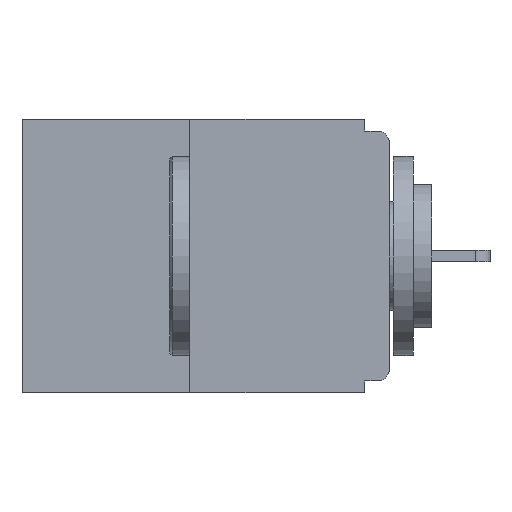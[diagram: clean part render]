
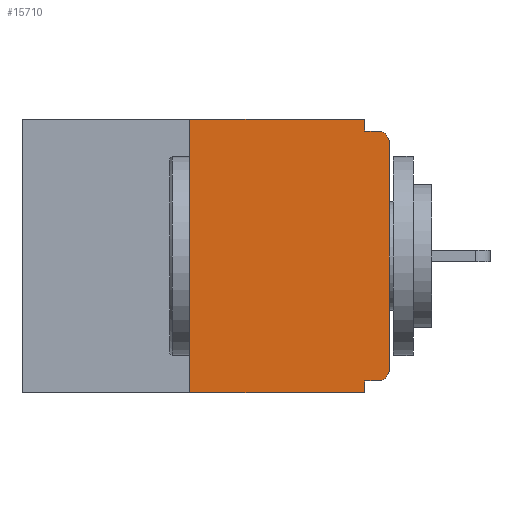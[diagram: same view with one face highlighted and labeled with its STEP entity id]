
A CAD part, left-side view. The second image highlights one B-rep face of the part: STEP entity #15710.
In plain terms, the highlighted planar face has unit normal (-1, 0, 0).
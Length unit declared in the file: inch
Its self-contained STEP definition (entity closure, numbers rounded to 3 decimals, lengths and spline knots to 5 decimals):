
#80 = VECTOR ( 'NONE', #3556, 39.37008 ) ;
#106 = EDGE_CURVE ( 'NONE', #14597, #6635, #15240, .T. ) ;
#530 = CARTESIAN_POINT ( 'NONE',  ( 0., 0.031, -0.343 ) ) ;
#645 = DIRECTION ( 'NONE',  ( 0., -1., 0. ) ) ;
#669 = VECTOR ( 'NONE', #9693, 39.37008 ) ;
#735 = VERTEX_POINT ( 'NONE', #10886 ) ;
#1963 = VERTEX_POINT ( 'NONE', #6756 ) ;
#2174 = CARTESIAN_POINT ( 'NONE',  ( 0., 0.031, -0.343 ) ) ;
#2885 = ORIENTED_EDGE ( 'NONE', *, *, #7124, .T. ) ;
#2951 = CARTESIAN_POINT ( 'NONE',  ( 0., 0.031, 0. ) ) ;
#3528 = EDGE_CURVE ( 'NONE', #10391, #17721, #3799, .T. ) ;
#3556 = DIRECTION ( 'NONE',  ( 0., -1., 0. ) ) ;
#3703 = DIRECTION ( 'NONE',  ( 0., 0., -1. ) ) ;
#3710 = LINE ( 'NONE', #10518, #11181 ) ;
#3799 = LINE ( 'NONE', #8110, #669 ) ;
#3952 = LINE ( 'NONE', #2951, #19208 ) ;
#4292 = VERTEX_POINT ( 'NONE', #530 ) ;
#4637 = LINE ( 'NONE', #11013, #80 ) ;
#4674 = DIRECTION ( 'NONE',  ( 0., 0., -1. ) ) ;
#4984 = ORIENTED_EDGE ( 'NONE', *, *, #16975, .F. ) ;
#5549 = AXIS2_PLACEMENT_3D ( 'NONE', #8939, #8842, #8495 ) ;
#6229 = VERTEX_POINT ( 'NONE', #10614 ) ;
#6635 = VERTEX_POINT ( 'NONE', #9253 ) ;
#6756 = CARTESIAN_POINT ( 'NONE',  ( 0., 0., -0.313 ) ) ;
#6788 = VECTOR ( 'NONE', #645, 39.37008 ) ;
#6792 = CARTESIAN_POINT ( 'NONE',  ( 0., 0.031, 0. ) ) ;
#6859 = ORIENTED_EDGE ( 'NONE', *, *, #19126, .T. ) ;
#6990 = CARTESIAN_POINT ( 'NONE',  ( 0., 0.25, 0. ) ) ;
#6999 = VECTOR ( 'NONE', #8473, 39.37008 ) ;
#7124 = EDGE_CURVE ( 'NONE', #10391, #1963, #13914, .T. ) ;
#7157 = LINE ( 'NONE', #9190, #17607 ) ;
#7274 = CARTESIAN_POINT ( 'NONE',  ( 0., 0.031, -0.328 ) ) ;
#7307 = ORIENTED_EDGE ( 'NONE', *, *, #106, .T. ) ;
#7962 = EDGE_LOOP ( 'NONE', ( #16405, #4984, #13426, #13890, #14345, #2885, #6859, #7307, #15253, #19100 ) ) ;
#8110 = CARTESIAN_POINT ( 'NONE',  ( 0., 0., -0.328 ) ) ;
#8422 = AXIS2_PLACEMENT_3D ( 'NONE', #12131, #13645, #4674 ) ;
#8466 = VERTEX_POINT ( 'NONE', #6792 ) ;
#8473 = DIRECTION ( 'NONE',  ( 0., 0., 1. ) ) ;
#8495 = DIRECTION ( 'NONE',  ( 0., 0., -1. ) ) ;
#8534 = CARTESIAN_POINT ( 'NONE',  ( 0., 0.015, -0.328 ) ) ;
#8842 = DIRECTION ( 'NONE',  ( -1., 0., 0. ) ) ;
#8939 = CARTESIAN_POINT ( 'NONE',  ( 0., 0.015, -0.03 ) ) ;
#9190 = CARTESIAN_POINT ( 'NONE',  ( 0., 0., 0. ) ) ;
#9253 = CARTESIAN_POINT ( 'NONE',  ( 0., 0.015, -0.015 ) ) ;
#9652 = CARTESIAN_POINT ( 'NONE',  ( 0., 0., -0.015 ) ) ;
#9693 = DIRECTION ( 'NONE',  ( 0., 1., 0. ) ) ;
#10391 = VERTEX_POINT ( 'NONE', #8534 ) ;
#10518 = CARTESIAN_POINT ( 'NONE',  ( 0., 0.46, -0.343 ) ) ;
#10614 = CARTESIAN_POINT ( 'NONE',  ( 0., 0.25, 0. ) ) ;
#10733 = CARTESIAN_POINT ( 'NONE',  ( 0., 0.031, -0.015 ) ) ;
#10886 = CARTESIAN_POINT ( 'NONE',  ( 0., 0.25, -0.343 ) ) ;
#11011 = LINE ( 'NONE', #6990, #6999 ) ;
#11013 = CARTESIAN_POINT ( 'NONE',  ( 0., 0.46, 0. ) ) ;
#11181 = VECTOR ( 'NONE', #16424, 39.37008 ) ;
#11700 = VECTOR ( 'NONE', #3703, 39.37008 ) ;
#11924 = EDGE_CURVE ( 'NONE', #17721, #4292, #16095, .T. ) ;
#12131 = CARTESIAN_POINT ( 'NONE',  ( 0., 0.46, 0. ) ) ;
#13426 = ORIENTED_EDGE ( 'NONE', *, *, #19044, .T. ) ;
#13645 = DIRECTION ( 'NONE',  ( 1., 0., 0. ) ) ;
#13684 = CARTESIAN_POINT ( 'NONE',  ( 0., 0., -0.03 ) ) ;
#13820 = LINE ( 'NONE', #9652, #6788 ) ;
#13890 = ORIENTED_EDGE ( 'NONE', *, *, #11924, .F. ) ;
#13914 = CIRCLE ( 'NONE', #14999, 0.015 ) ;
#14345 = ORIENTED_EDGE ( 'NONE', *, *, #3528, .F. ) ;
#14597 = VERTEX_POINT ( 'NONE', #13684 ) ;
#14999 = AXIS2_PLACEMENT_3D ( 'NONE', #17262, #17235, #17215 ) ;
#15240 = CIRCLE ( 'NONE', #5549, 0.015 ) ;
#15253 = ORIENTED_EDGE ( 'NONE', *, *, #17448, .F. ) ;
#15710 = ADVANCED_FACE ( 'NONE', ( #17957 ), #16521, .F. ) ;
#16095 = LINE ( 'NONE', #2174, #11700 ) ;
#16388 = VERTEX_POINT ( 'NONE', #10733 ) ;
#16405 = ORIENTED_EDGE ( 'NONE', *, *, #18597, .F. ) ;
#16424 = DIRECTION ( 'NONE',  ( 0., -1., 0. ) ) ;
#16521 = PLANE ( 'NONE',  #8422 ) ;
#16682 = DIRECTION ( 'NONE',  ( 0., 0., 1. ) ) ;
#16975 = EDGE_CURVE ( 'NONE', #735, #6229, #11011, .T. ) ;
#17215 = DIRECTION ( 'NONE',  ( 0., 0., -1. ) ) ;
#17235 = DIRECTION ( 'NONE',  ( -1., 0., 0. ) ) ;
#17262 = CARTESIAN_POINT ( 'NONE',  ( 0., 0.015, -0.313 ) ) ;
#17448 = EDGE_CURVE ( 'NONE', #16388, #6635, #13820, .T. ) ;
#17607 = VECTOR ( 'NONE', #16682, 39.37008 ) ;
#17721 = VERTEX_POINT ( 'NONE', #7274 ) ;
#17828 = DIRECTION ( 'NONE',  ( 0., 0., -1. ) ) ;
#17957 = FACE_OUTER_BOUND ( 'NONE', #7962, .T. ) ;
#18406 = EDGE_CURVE ( 'NONE', #8466, #16388, #3952, .T. ) ;
#18597 = EDGE_CURVE ( 'NONE', #6229, #8466, #4637, .T. ) ;
#19044 = EDGE_CURVE ( 'NONE', #735, #4292, #3710, .T. ) ;
#19100 = ORIENTED_EDGE ( 'NONE', *, *, #18406, .F. ) ;
#19126 = EDGE_CURVE ( 'NONE', #1963, #14597, #7157, .T. ) ;
#19208 = VECTOR ( 'NONE', #17828, 39.37008 ) ;
